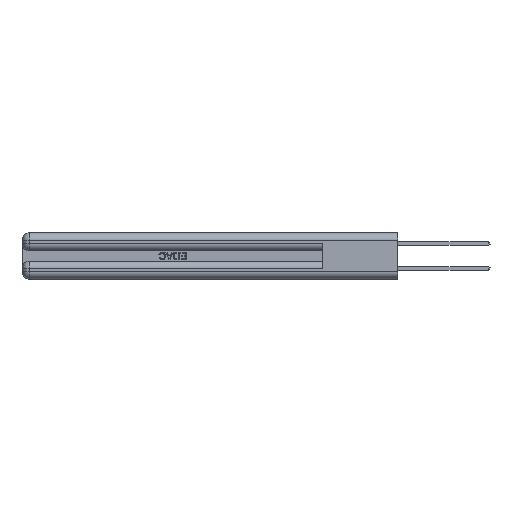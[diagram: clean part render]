
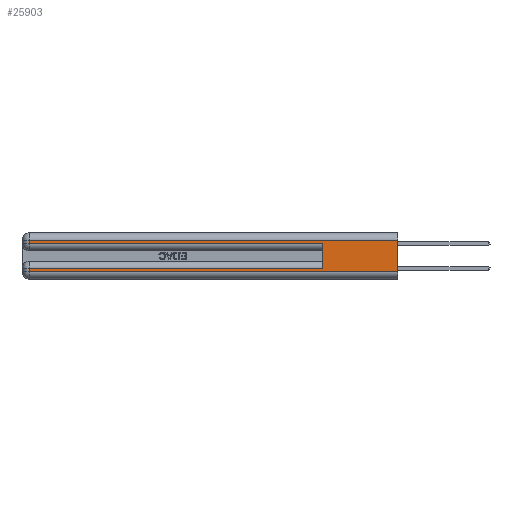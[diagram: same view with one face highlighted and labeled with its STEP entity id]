
A CAD part, left-side view. The second image highlights one B-rep face of the part: STEP entity #25903.
In plain terms, the highlighted planar face has unit normal (-1, 0, 0).
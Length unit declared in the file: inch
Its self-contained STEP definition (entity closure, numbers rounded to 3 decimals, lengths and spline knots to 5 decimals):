
#778 = CARTESIAN_POINT ( 'NONE',  ( 0., 0.6, 0.085 ) ) ;
#1159 = LINE ( 'NONE', #36520, #39221 ) ;
#1996 = EDGE_CURVE ( 'NONE', #46565, #30770, #25492, .T. ) ;
#2519 = LINE ( 'NONE', #8107, #41739 ) ;
#2667 = PLANE ( 'NONE',  #21257 ) ;
#3832 = CARTESIAN_POINT ( 'NONE',  ( 0., 2.94, 0.06 ) ) ;
#4250 = VECTOR ( 'NONE', #23686, 39.37008 ) ;
#4695 = DIRECTION ( 'NONE',  ( 0., 0., -1. ) ) ;
#6492 = DIRECTION ( 'NONE',  ( 0., 0., -1. ) ) ;
#6509 = EDGE_CURVE ( 'NONE', #31440, #10609, #40539, .T. ) ;
#6731 = ORIENTED_EDGE ( 'NONE', *, *, #6509, .T. ) ;
#7473 = CARTESIAN_POINT ( 'NONE',  ( 0., 0., 0.31 ) ) ;
#7651 = CARTESIAN_POINT ( 'NONE',  ( 0., 0., 0.06 ) ) ;
#7822 = ORIENTED_EDGE ( 'NONE', *, *, #1996, .T. ) ;
#7827 = EDGE_CURVE ( 'NONE', #30770, #11681, #39642, .T. ) ;
#8107 = CARTESIAN_POINT ( 'NONE',  ( 0., 0., 0.285 ) ) ;
#9337 = FACE_OUTER_BOUND ( 'NONE', #40044, .T. ) ;
#10609 = VERTEX_POINT ( 'NONE', #16416 ) ;
#11681 = VERTEX_POINT ( 'NONE', #3832 ) ;
#12151 = ORIENTED_EDGE ( 'NONE', *, *, #19507, .T. ) ;
#13518 = LINE ( 'NONE', #27065, #32490 ) ;
#13940 = CARTESIAN_POINT ( 'NONE',  ( 0., 0.6, 0.145 ) ) ;
#15142 = CARTESIAN_POINT ( 'NONE',  ( 0., 0., 0.085 ) ) ;
#16039 = CARTESIAN_POINT ( 'NONE',  ( 0., 2.94, 0.37 ) ) ;
#16416 = CARTESIAN_POINT ( 'NONE',  ( 0., 2.94, 0.285 ) ) ;
#17744 = DIRECTION ( 'NONE',  ( 0., 0., 1. ) ) ;
#18783 = EDGE_CURVE ( 'NONE', #11681, #32413, #44633, .T. ) ;
#19046 = ORIENTED_EDGE ( 'NONE', *, *, #22255, .F. ) ;
#19507 = EDGE_CURVE ( 'NONE', #22144, #31440, #1159, .T. ) ;
#20381 = VECTOR ( 'NONE', #45481, 39.37008 ) ;
#21257 = AXIS2_PLACEMENT_3D ( 'NONE', #29080, #29246, #6492 ) ;
#22144 = VERTEX_POINT ( 'NONE', #7473 ) ;
#22255 = EDGE_CURVE ( 'NONE', #22144, #32413, #13518, .T. ) ;
#22746 = DIRECTION ( 'NONE',  ( 0., 1., 0. ) ) ;
#23686 = DIRECTION ( 'NONE',  ( 0., -1., 0. ) ) ;
#24335 = VERTEX_POINT ( 'NONE', #42663 ) ;
#24400 = CARTESIAN_POINT ( 'NONE',  ( 0., 2.94, 0.085 ) ) ;
#24945 = ORIENTED_EDGE ( 'NONE', *, *, #7827, .T. ) ;
#25108 = ORIENTED_EDGE ( 'NONE', *, *, #28594, .T. ) ;
#25492 = LINE ( 'NONE', #15142, #44458 ) ;
#25903 = ADVANCED_FACE ( 'NONE', ( #9337 ), #2667, .F. ) ;
#27030 = EDGE_CURVE ( 'NONE', #46565, #24335, #41302, .T. ) ;
#27065 = CARTESIAN_POINT ( 'NONE',  ( 0., 0., 0.37 ) ) ;
#28275 = ORIENTED_EDGE ( 'NONE', *, *, #27030, .F. ) ;
#28594 = EDGE_CURVE ( 'NONE', #10609, #24335, #2519, .T. ) ;
#28894 = DIRECTION ( 'NONE',  ( 0., 1., 0. ) ) ;
#29080 = CARTESIAN_POINT ( 'NONE',  ( 0., 0., 0.37 ) ) ;
#29246 = DIRECTION ( 'NONE',  ( 1., 0., 0. ) ) ;
#30394 = CARTESIAN_POINT ( 'NONE',  ( 0., 2.94, 0.37 ) ) ;
#30770 = VERTEX_POINT ( 'NONE', #24400 ) ;
#30872 = DIRECTION ( 'NONE',  ( 0., -1., 0. ) ) ;
#30881 = DIRECTION ( 'NONE',  ( 0., 0., -1. ) ) ;
#31440 = VERTEX_POINT ( 'NONE', #40286 ) ;
#32413 = VERTEX_POINT ( 'NONE', #7651 ) ;
#32490 = VECTOR ( 'NONE', #30881, 39.37008 ) ;
#33464 = ORIENTED_EDGE ( 'NONE', *, *, #18783, .T. ) ;
#36520 = CARTESIAN_POINT ( 'NONE',  ( 0., 0., 0.31 ) ) ;
#39221 = VECTOR ( 'NONE', #28894, 39.37008 ) ;
#39642 = LINE ( 'NONE', #16039, #48528 ) ;
#40044 = EDGE_LOOP ( 'NONE', ( #19046, #12151, #6731, #25108, #28275, #7822, #24945, #33464 ) ) ;
#40286 = CARTESIAN_POINT ( 'NONE',  ( 0., 2.94, 0.31 ) ) ;
#40539 = LINE ( 'NONE', #30394, #20381 ) ;
#41302 = LINE ( 'NONE', #13940, #42497 ) ;
#41739 = VECTOR ( 'NONE', #30872, 39.37008 ) ;
#42497 = VECTOR ( 'NONE', #17744, 39.37008 ) ;
#42663 = CARTESIAN_POINT ( 'NONE',  ( 0., 0.6, 0.285 ) ) ;
#44458 = VECTOR ( 'NONE', #22746, 39.37008 ) ;
#44633 = LINE ( 'NONE', #46244, #4250 ) ;
#45481 = DIRECTION ( 'NONE',  ( 0., 0., -1. ) ) ;
#46244 = CARTESIAN_POINT ( 'NONE',  ( 0., 0., 0.06 ) ) ;
#46565 = VERTEX_POINT ( 'NONE', #778 ) ;
#48528 = VECTOR ( 'NONE', #4695, 39.37008 ) ;
